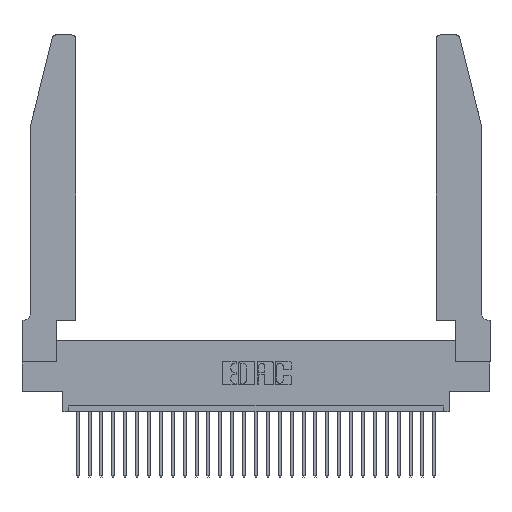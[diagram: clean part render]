
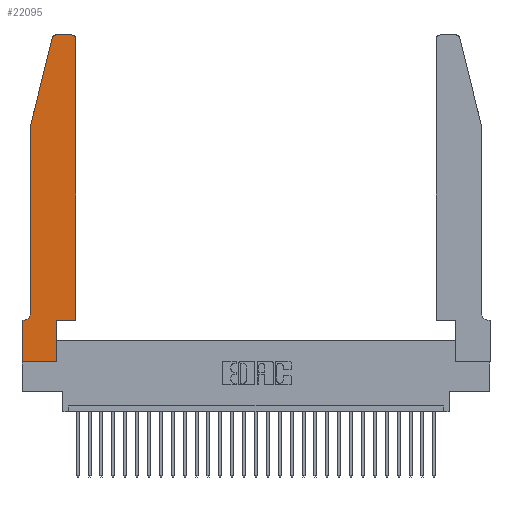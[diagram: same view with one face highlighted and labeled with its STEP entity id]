
A CAD part, top view. The second image highlights one B-rep face of the part: STEP entity #22095.
In plain terms, the highlighted planar face has unit normal (0, 0, 1).
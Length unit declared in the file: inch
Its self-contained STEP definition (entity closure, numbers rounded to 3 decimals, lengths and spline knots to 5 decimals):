
#192 = VECTOR ( 'NONE', #20795, 39.37008 ) ;
#259 = DIRECTION ( 'NONE',  ( -1., 0., 0. ) ) ;
#482 = CARTESIAN_POINT ( 'NONE',  ( 0.4505, 0.35, 0.37 ) ) ;
#555 = ORIENTED_EDGE ( 'NONE', *, *, #28805, .T. ) ;
#1009 = CARTESIAN_POINT ( 'NONE',  ( 0.4205, 2.75, 0.37 ) ) ;
#1044 = DIRECTION ( 'NONE',  ( 1., 0., 0. ) ) ;
#1547 = ORIENTED_EDGE ( 'NONE', *, *, #6166, .T. ) ;
#2234 = ORIENTED_EDGE ( 'NONE', *, *, #28196, .T. ) ;
#2263 = CARTESIAN_POINT ( 'NONE',  ( 0.0755, 2., 0.37 ) ) ;
#2305 = CARTESIAN_POINT ( 'NONE',  ( 0., 0.35, 0.37 ) ) ;
#2503 = EDGE_CURVE ( 'NONE', #25874, #28250, #25085, .T. ) ;
#2508 = VERTEX_POINT ( 'NONE', #14317 ) ;
#2965 = CARTESIAN_POINT ( 'NONE',  ( 0.0755, 0.35, 0.37 ) ) ;
#3304 = LINE ( 'NONE', #25791, #27004 ) ;
#3320 = CARTESIAN_POINT ( 'NONE',  ( 0., 0., 0.37 ) ) ;
#3647 = CARTESIAN_POINT ( 'NONE',  ( 0.0055, 0.42, 0.37 ) ) ;
#4241 = DIRECTION ( 'NONE',  ( 0., 0., -1. ) ) ;
#5189 = EDGE_CURVE ( 'NONE', #9295, #15854, #27292, .T. ) ;
#5202 = DIRECTION ( 'NONE',  ( 0., 0., 1. ) ) ;
#5305 = CARTESIAN_POINT ( 'NONE',  ( 0.284, 2.72, 0.37 ) ) ;
#5557 = EDGE_CURVE ( 'NONE', #15854, #7597, #27974, .T. ) ;
#5712 = VERTEX_POINT ( 'NONE', #21298 ) ;
#6166 = EDGE_CURVE ( 'NONE', #5712, #27168, #18587, .T. ) ;
#6653 = LINE ( 'NONE', #18935, #28161 ) ;
#7597 = VERTEX_POINT ( 'NONE', #25578 ) ;
#7766 = LINE ( 'NONE', #20981, #192 ) ;
#8076 = CARTESIAN_POINT ( 'NONE',  ( 0.2865, 0.35, 0.37 ) ) ;
#8189 = EDGE_CURVE ( 'NONE', #13889, #5712, #7766, .T. ) ;
#8337 = LINE ( 'NONE', #24439, #27353 ) ;
#8915 = DIRECTION ( 'NONE',  ( -1., 0., 0. ) ) ;
#9001 = VERTEX_POINT ( 'NONE', #3320 ) ;
#9059 = LINE ( 'NONE', #20248, #11197 ) ;
#9177 = DIRECTION ( 'NONE',  ( 1., 0., 0. ) ) ;
#9229 = CARTESIAN_POINT ( 'NONE',  ( 0.2865, 0., 0.37 ) ) ;
#9295 = VERTEX_POINT ( 'NONE', #9229 ) ;
#9461 = CARTESIAN_POINT ( 'NONE',  ( 0.4505, 2.72, 0.37 ) ) ;
#9507 = CARTESIAN_POINT ( 'NONE',  ( 0.2865, 0.35, 0.37 ) ) ;
#9633 = FACE_OUTER_BOUND ( 'NONE', #19016, .T. ) ;
#9859 = DIRECTION ( 'NONE',  ( 1., 0., 0. ) ) ;
#10363 = LINE ( 'NONE', #21613, #24343 ) ;
#10395 = VECTOR ( 'NONE', #27689, 39.37008 ) ;
#10630 = ORIENTED_EDGE ( 'NONE', *, *, #19310, .T. ) ;
#11197 = VECTOR ( 'NONE', #27196, 39.37008 ) ;
#11664 = DIRECTION ( 'NONE',  ( -1., 0., 0. ) ) ;
#11847 = ORIENTED_EDGE ( 'NONE', *, *, #5557, .T. ) ;
#11939 = ORIENTED_EDGE ( 'NONE', *, *, #2503, .T. ) ;
#12294 = AXIS2_PLACEMENT_3D ( 'NONE', #3647, #4241, #8915 ) ;
#13074 = ORIENTED_EDGE ( 'NONE', *, *, #25900, .T. ) ;
#13889 = VERTEX_POINT ( 'NONE', #2263 ) ;
#14261 = AXIS2_PLACEMENT_3D ( 'NONE', #5305, #5202, #16831 ) ;
#14317 = CARTESIAN_POINT ( 'NONE',  ( 0., 0.35, 0.37 ) ) ;
#14508 = DIRECTION ( 'NONE',  ( 0., -1., 0. ) ) ;
#14531 = VERTEX_POINT ( 'NONE', #16179 ) ;
#15051 = ORIENTED_EDGE ( 'NONE', *, *, #18987, .T. ) ;
#15117 = EDGE_CURVE ( 'NONE', #7597, #25874, #9059, .T. ) ;
#15197 = DIRECTION ( 'NONE',  ( -0.239, -0.971, 0. ) ) ;
#15381 = CARTESIAN_POINT ( 'NONE',  ( 0.0055, 0.35, 0.37 ) ) ;
#15854 = VERTEX_POINT ( 'NONE', #9507 ) ;
#16179 = CARTESIAN_POINT ( 'NONE',  ( 0.284, 2.75, 0.37 ) ) ;
#16352 = ORIENTED_EDGE ( 'NONE', *, *, #24122, .T. ) ;
#16370 = CARTESIAN_POINT ( 'NONE',  ( 0.25487, 2.72718, 0.37 ) ) ;
#16406 = VERTEX_POINT ( 'NONE', #16370 ) ;
#16607 = AXIS2_PLACEMENT_3D ( 'NONE', #2305, #22790, #9177 ) ;
#16831 = DIRECTION ( 'NONE',  ( 1., 0., 0. ) ) ;
#16905 = CIRCLE ( 'NONE', #14261, 0.03 ) ;
#16926 = VECTOR ( 'NONE', #259, 39.37008 ) ;
#17322 = ORIENTED_EDGE ( 'NONE', *, *, #5189, .T. ) ;
#17896 = ORIENTED_EDGE ( 'NONE', *, *, #15117, .T. ) ;
#17949 = PLANE ( 'NONE',  #16607 ) ;
#18587 = CIRCLE ( 'NONE', #12294, 0.07 ) ;
#18889 = CARTESIAN_POINT ( 'NONE',  ( 0.4205, 2.72, 0.37 ) ) ;
#18935 = CARTESIAN_POINT ( 'NONE',  ( 0.2605, 2.75, 0.37 ) ) ;
#18987 = EDGE_CURVE ( 'NONE', #27168, #2508, #24853, .T. ) ;
#19016 = EDGE_LOOP ( 'NONE', ( #13074, #555, #10630, #28438, #1547, #15051, #16352, #2234, #17322, #11847, #17896, #11939 ) ) ;
#19310 = EDGE_CURVE ( 'NONE', #16406, #13889, #8337, .T. ) ;
#20248 = CARTESIAN_POINT ( 'NONE',  ( 0.4505, 0.35, 0.37 ) ) ;
#20795 = DIRECTION ( 'NONE',  ( 0., -1., 0. ) ) ;
#20981 = CARTESIAN_POINT ( 'NONE',  ( 0.0755, 2., 0.37 ) ) ;
#21298 = CARTESIAN_POINT ( 'NONE',  ( 0.0755, 0.42, 0.37 ) ) ;
#21514 = DIRECTION ( 'NONE',  ( 0., 0., 1. ) ) ;
#21613 = CARTESIAN_POINT ( 'NONE',  ( 0., 0., 0.37 ) ) ;
#22095 = ADVANCED_FACE ( 'NONE', ( #9633 ), #17949, .T. ) ;
#22237 = AXIS2_PLACEMENT_3D ( 'NONE', #18889, #21514, #1044 ) ;
#22790 = DIRECTION ( 'NONE',  ( 0., 0., 1. ) ) ;
#24108 = DIRECTION ( 'NONE',  ( 0., 1., 0. ) ) ;
#24122 = EDGE_CURVE ( 'NONE', #2508, #9001, #10363, .T. ) ;
#24343 = VECTOR ( 'NONE', #14508, 39.37008 ) ;
#24414 = VECTOR ( 'NONE', #24108, 39.37008 ) ;
#24439 = CARTESIAN_POINT ( 'NONE',  ( 0.0755, 2., 0.37 ) ) ;
#24853 = LINE ( 'NONE', #2965, #16926 ) ;
#25085 = CIRCLE ( 'NONE', #22237, 0.03 ) ;
#25578 = CARTESIAN_POINT ( 'NONE',  ( 0.4505, 0.35, 0.37 ) ) ;
#25791 = CARTESIAN_POINT ( 'NONE',  ( 0., 0., 0.37 ) ) ;
#25874 = VERTEX_POINT ( 'NONE', #9461 ) ;
#25900 = EDGE_CURVE ( 'NONE', #28250, #14531, #6653, .T. ) ;
#27004 = VECTOR ( 'NONE', #9859, 39.37008 ) ;
#27168 = VERTEX_POINT ( 'NONE', #15381 ) ;
#27196 = DIRECTION ( 'NONE',  ( 0., 1., 0. ) ) ;
#27292 = LINE ( 'NONE', #8076, #24414 ) ;
#27353 = VECTOR ( 'NONE', #15197, 39.37008 ) ;
#27689 = DIRECTION ( 'NONE',  ( 1., 0., 0. ) ) ;
#27974 = LINE ( 'NONE', #482, #10395 ) ;
#28161 = VECTOR ( 'NONE', #11664, 39.37008 ) ;
#28196 = EDGE_CURVE ( 'NONE', #9001, #9295, #3304, .T. ) ;
#28250 = VERTEX_POINT ( 'NONE', #1009 ) ;
#28438 = ORIENTED_EDGE ( 'NONE', *, *, #8189, .T. ) ;
#28805 = EDGE_CURVE ( 'NONE', #14531, #16406, #16905, .T. ) ;
